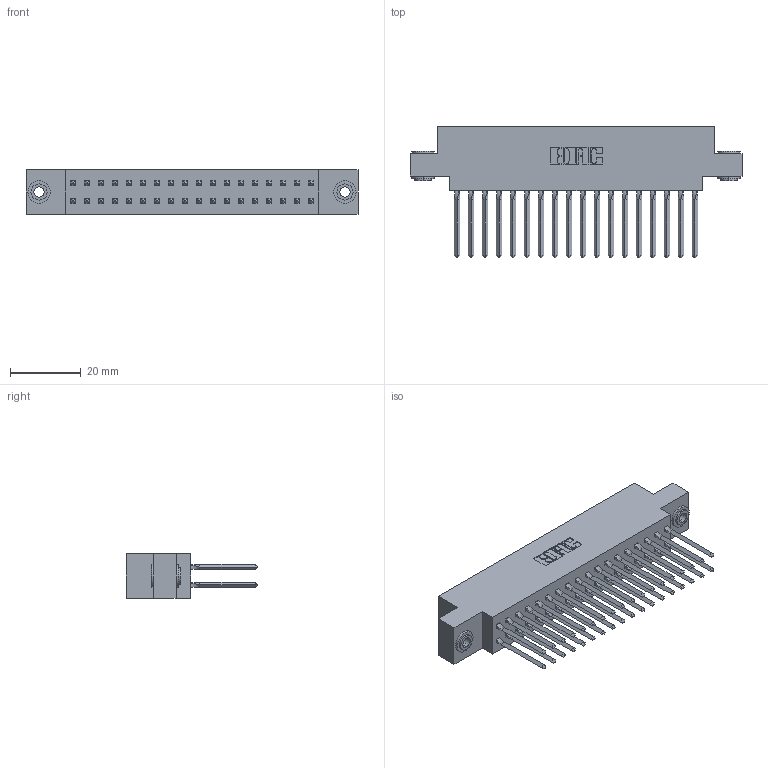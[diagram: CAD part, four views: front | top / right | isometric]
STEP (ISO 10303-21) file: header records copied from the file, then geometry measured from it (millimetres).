
FILE_DESCRIPTION (( 'STEP AP203' ), '1' );
FILE_NAME ('317-036-540-803.STEP', '2020-02-27T22:44:46', ( '' ), ( '' ), 'SwSTEP 2.0', 'SolidWorks 2016', '' );
FILE_SCHEMA (( 'CONFIG_CONTROL_DESIGN' ));
Length unit declared in the file: inch
Products named in the file (4): 317 Part_.156 Dia - TH; 317-036-540-803; 317-290-001_540; 345-250-002_345-250-002-102
Assembly tree (39 placements, depth 2):
  317-036-540-803
    317 Part_.156 Dia - TH
    317-290-001_540  x36
    345-250-002_345-250-002-102  x2
Bounding box: 94.03 x 37.34 x 12.7 mm (x, y, z)
Volume: 14989.2 mm3; surface area: 21654.4 mm2
Topology: 39 solids, 39 shells, 3344 faces, 9243 edges, 5954 vertices
Faces by surface type: plane 2696, cylinder 496, bspline 144, cone 8
Entity records: 30017 total; most frequent: CARTESIAN_POINT 5618, ORIENTED_EDGE 5110, DIRECTION 4307, EDGE_CURVE 2555, VECTOR 2275, LINE 2275, VERTEX_POINT 1695, AXIS2_PLACEMENT_3D 1016
